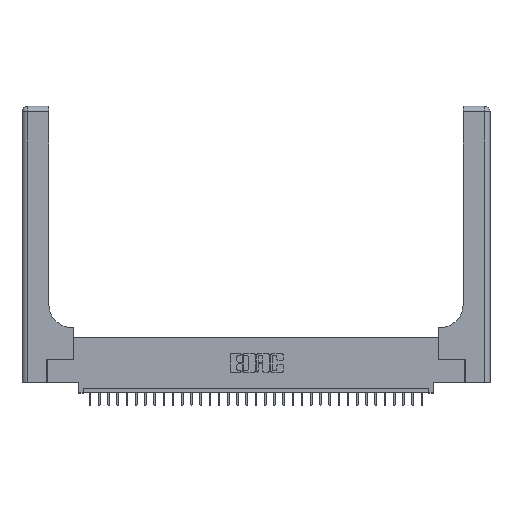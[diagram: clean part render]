
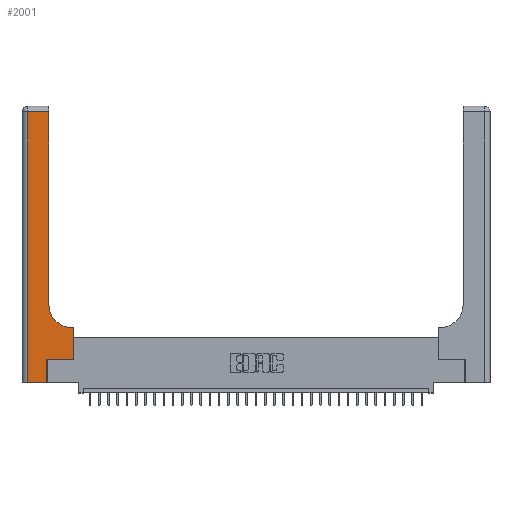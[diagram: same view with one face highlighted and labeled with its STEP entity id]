
A CAD part, top view. The second image highlights one B-rep face of the part: STEP entity #2001.
In plain terms, the highlighted planar face has unit normal (0, 0, 1).
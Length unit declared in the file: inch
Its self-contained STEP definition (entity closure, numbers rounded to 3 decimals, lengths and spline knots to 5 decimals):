
#237 = VECTOR ( 'NONE', #3465, 39.37008 ) ;
#870 = EDGE_CURVE ( 'NONE', #4022, #20775, #11323, .T. ) ;
#1907 = VERTEX_POINT ( 'NONE', #32293 ) ;
#1981 = ORIENTED_EDGE ( 'NONE', *, *, #21822, .T. ) ;
#2001 = ADVANCED_FACE ( 'NONE', ( #9122 ), #29890, .F. ) ;
#2636 = CARTESIAN_POINT ( 'NONE',  ( 0.5415, 0.6, 0.37 ) ) ;
#3003 = VERTEX_POINT ( 'NONE', #21305 ) ;
#3465 = DIRECTION ( 'NONE',  ( 0., 1., 0. ) ) ;
#4022 = VERTEX_POINT ( 'NONE', #13844 ) ;
#4367 = DIRECTION ( 'NONE',  ( -1., 0., 0. ) ) ;
#4720 = VERTEX_POINT ( 'NONE', #2636 ) ;
#4839 = ORIENTED_EDGE ( 'NONE', *, *, #870, .T. ) ;
#4961 = EDGE_LOOP ( 'NONE', ( #24189, #4839, #26959, #1981, #13448, #20688, #18220, #20282, #19782 ) ) ;
#5546 = DIRECTION ( 'NONE',  ( 0., 0., -1. ) ) ;
#5718 = CARTESIAN_POINT ( 'NONE',  ( 0.2915, 3., 0.37 ) ) ;
#6733 = DIRECTION ( 'NONE',  ( -1., 0., 0. ) ) ;
#7458 = EDGE_CURVE ( 'NONE', #1907, #3003, #9907, .T. ) ;
#8805 = CARTESIAN_POINT ( 'NONE',  ( 0.2915, 0.85, 0.37 ) ) ;
#9122 = FACE_OUTER_BOUND ( 'NONE', #4961, .T. ) ;
#9907 = LINE ( 'NONE', #20358, #28831 ) ;
#10892 = VECTOR ( 'NONE', #32255, 39.37008 ) ;
#11323 = LINE ( 'NONE', #21766, #10892 ) ;
#12255 = VECTOR ( 'NONE', #27630, 39.37008 ) ;
#13448 = ORIENTED_EDGE ( 'NONE', *, *, #7458, .T. ) ;
#13844 = CARTESIAN_POINT ( 'NONE',  ( 0.2915, 2.94, 0.37 ) ) ;
#14639 = LINE ( 'NONE', #20113, #29994 ) ;
#14707 = DIRECTION ( 'NONE',  ( 0., 1., 0. ) ) ;
#15177 = CARTESIAN_POINT ( 'NONE',  ( 0.5585, 0.25, 0.37 ) ) ;
#15258 = EDGE_CURVE ( 'NONE', #4720, #24730, #29561, .T. ) ;
#15313 = AXIS2_PLACEMENT_3D ( 'NONE', #24392, #5546, #27154 ) ;
#15412 = CARTESIAN_POINT ( 'NONE',  ( 0., 0., 0.37 ) ) ;
#15508 = VERTEX_POINT ( 'NONE', #28506 ) ;
#15575 = VECTOR ( 'NONE', #26264, 39.37008 ) ;
#15745 = LINE ( 'NONE', #15412, #19904 ) ;
#15787 = CARTESIAN_POINT ( 'NONE',  ( 0.269, 0.25, 0.37 ) ) ;
#16642 = LINE ( 'NONE', #21619, #237 ) ;
#16900 = VECTOR ( 'NONE', #19396, 39.37008 ) ;
#16995 = DIRECTION ( 'NONE',  ( 0., 0., -1. ) ) ;
#18220 = ORIENTED_EDGE ( 'NONE', *, *, #22903, .T. ) ;
#19396 = DIRECTION ( 'NONE',  ( 0., 1., 0. ) ) ;
#19523 = EDGE_CURVE ( 'NONE', #20775, #15508, #27964, .T. ) ;
#19552 = CARTESIAN_POINT ( 'NONE',  ( 0., 3., 0.37 ) ) ;
#19782 = ORIENTED_EDGE ( 'NONE', *, *, #15258, .T. ) ;
#19904 = VECTOR ( 'NONE', #25729, 39.37008 ) ;
#20113 = CARTESIAN_POINT ( 'NONE',  ( 0.2915, 0.6, 0.37 ) ) ;
#20282 = ORIENTED_EDGE ( 'NONE', *, *, #29176, .T. ) ;
#20358 = CARTESIAN_POINT ( 'NONE',  ( 0.269, 0., 0.37 ) ) ;
#20688 = ORIENTED_EDGE ( 'NONE', *, *, #22780, .T. ) ;
#20775 = VERTEX_POINT ( 'NONE', #24617 ) ;
#21305 = CARTESIAN_POINT ( 'NONE',  ( 0.269, 0.25, 0.37 ) ) ;
#21575 = VERTEX_POINT ( 'NONE', #26433 ) ;
#21619 = CARTESIAN_POINT ( 'NONE',  ( 0.5585, 0.25, 0.37 ) ) ;
#21766 = CARTESIAN_POINT ( 'NONE',  ( 0., 2.94, 0.37 ) ) ;
#21822 = EDGE_CURVE ( 'NONE', #15508, #1907, #15745, .T. ) ;
#22780 = EDGE_CURVE ( 'NONE', #3003, #28654, #28855, .T. ) ;
#22903 = EDGE_CURVE ( 'NONE', #28654, #21575, #16642, .T. ) ;
#24189 = ORIENTED_EDGE ( 'NONE', *, *, #30763, .T. ) ;
#24392 = CARTESIAN_POINT ( 'NONE',  ( 0.5415, 0.85, 0.37 ) ) ;
#24617 = CARTESIAN_POINT ( 'NONE',  ( 0.06, 2.94, 0.37 ) ) ;
#24730 = VERTEX_POINT ( 'NONE', #8805 ) ;
#25729 = DIRECTION ( 'NONE',  ( 1., 0., 0. ) ) ;
#26264 = DIRECTION ( 'NONE',  ( 1., 0., 0. ) ) ;
#26433 = CARTESIAN_POINT ( 'NONE',  ( 0.5585, 0.6, 0.37 ) ) ;
#26738 = AXIS2_PLACEMENT_3D ( 'NONE', #19552, #16995, #6733 ) ;
#26959 = ORIENTED_EDGE ( 'NONE', *, *, #19523, .T. ) ;
#27154 = DIRECTION ( 'NONE',  ( 1., 0., 0. ) ) ;
#27630 = DIRECTION ( 'NONE',  ( 0., -1., 0. ) ) ;
#27964 = LINE ( 'NONE', #30876, #12255 ) ;
#28506 = CARTESIAN_POINT ( 'NONE',  ( 0.06, 0., 0.37 ) ) ;
#28654 = VERTEX_POINT ( 'NONE', #15177 ) ;
#28831 = VECTOR ( 'NONE', #14707, 39.37008 ) ;
#28855 = LINE ( 'NONE', #15787, #15575 ) ;
#29176 = EDGE_CURVE ( 'NONE', #21575, #4720, #14639, .T. ) ;
#29561 = CIRCLE ( 'NONE', #15313, 0.25 ) ;
#29890 = PLANE ( 'NONE',  #26738 ) ;
#29901 = LINE ( 'NONE', #5718, #16900 ) ;
#29994 = VECTOR ( 'NONE', #4367, 39.37008 ) ;
#30763 = EDGE_CURVE ( 'NONE', #24730, #4022, #29901, .T. ) ;
#30876 = CARTESIAN_POINT ( 'NONE',  ( 0.06, 3., 0.37 ) ) ;
#32255 = DIRECTION ( 'NONE',  ( -1., 0., 0. ) ) ;
#32293 = CARTESIAN_POINT ( 'NONE',  ( 0.269, 0., 0.37 ) ) ;
